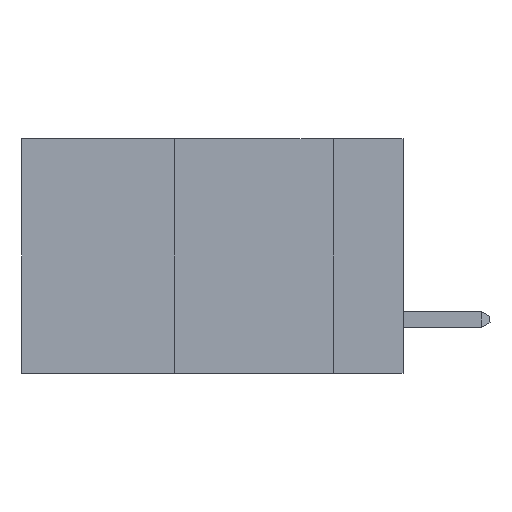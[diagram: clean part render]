
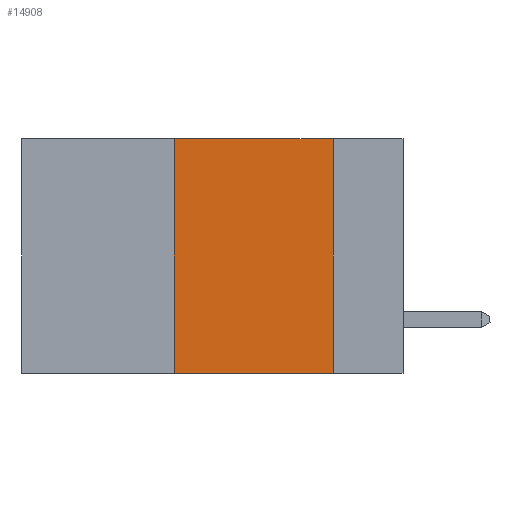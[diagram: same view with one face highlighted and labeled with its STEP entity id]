
A CAD part, left-side view. The second image highlights one B-rep face of the part: STEP entity #14908.
In plain terms, the highlighted planar face has unit normal (-1, 0, 0).
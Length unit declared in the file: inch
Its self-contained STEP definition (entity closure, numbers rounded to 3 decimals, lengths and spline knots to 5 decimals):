
#167 = AXIS2_PLACEMENT_3D ( 'NONE', #16502, #6060, #18195 ) ;
#634 = VECTOR ( 'NONE', #14794, 39.37008 ) ;
#663 = DIRECTION ( 'NONE',  ( 0., -1., 0. ) ) ;
#746 = CARTESIAN_POINT ( 'NONE',  ( 0., 0.6, -0.37 ) ) ;
#875 = ORIENTED_EDGE ( 'NONE', *, *, #21673, .F. ) ;
#2626 = VECTOR ( 'NONE', #20001, 39.37008 ) ;
#4092 = VECTOR ( 'NONE', #7222, 39.37008 ) ;
#4272 = LINE ( 'NONE', #746, #4816 ) ;
#4816 = VECTOR ( 'NONE', #663, 39.37008 ) ;
#5434 = CARTESIAN_POINT ( 'NONE',  ( 0., 0.6, 0. ) ) ;
#5677 = VERTEX_POINT ( 'NONE', #15932 ) ;
#5839 = LINE ( 'NONE', #6082, #634 ) ;
#6060 = DIRECTION ( 'NONE',  ( 1., 0., 0. ) ) ;
#6082 = CARTESIAN_POINT ( 'NONE',  ( 0., 0.36, 0. ) ) ;
#6743 = LINE ( 'NONE', #7911, #2626 ) ;
#7222 = DIRECTION ( 'NONE',  ( 0., -1., 0. ) ) ;
#7911 = CARTESIAN_POINT ( 'NONE',  ( 0., 0.11, 0. ) ) ;
#9155 = VERTEX_POINT ( 'NONE', #21210 ) ;
#10629 = VERTEX_POINT ( 'NONE', #21598 ) ;
#10779 = ORIENTED_EDGE ( 'NONE', *, *, #11926, .T. ) ;
#10820 = VERTEX_POINT ( 'NONE', #16890 ) ;
#11926 = EDGE_CURVE ( 'NONE', #9155, #10629, #4272, .T. ) ;
#14794 = DIRECTION ( 'NONE',  ( 0., 0., 1. ) ) ;
#14908 = ADVANCED_FACE ( 'NONE', ( #18569 ), #21575, .F. ) ;
#15932 = CARTESIAN_POINT ( 'NONE',  ( 0., 0.36, 0. ) ) ;
#16502 = CARTESIAN_POINT ( 'NONE',  ( 0., 0.6, 0. ) ) ;
#16565 = EDGE_CURVE ( 'NONE', #5677, #10820, #22486, .T. ) ;
#16890 = CARTESIAN_POINT ( 'NONE',  ( 0., 0.11, 0. ) ) ;
#18195 = DIRECTION ( 'NONE',  ( 0., 0., -1. ) ) ;
#18278 = ORIENTED_EDGE ( 'NONE', *, *, #20542, .F. ) ;
#18569 = FACE_OUTER_BOUND ( 'NONE', #20395, .T. ) ;
#18816 = ORIENTED_EDGE ( 'NONE', *, *, #16565, .F. ) ;
#20001 = DIRECTION ( 'NONE',  ( 0., 0., -1. ) ) ;
#20395 = EDGE_LOOP ( 'NONE', ( #18278, #18816, #875, #10779 ) ) ;
#20542 = EDGE_CURVE ( 'NONE', #10820, #10629, #6743, .T. ) ;
#21210 = CARTESIAN_POINT ( 'NONE',  ( 0., 0.36, -0.37 ) ) ;
#21575 = PLANE ( 'NONE',  #167 ) ;
#21598 = CARTESIAN_POINT ( 'NONE',  ( 0., 0.11, -0.37 ) ) ;
#21673 = EDGE_CURVE ( 'NONE', #9155, #5677, #5839, .T. ) ;
#22486 = LINE ( 'NONE', #5434, #4092 ) ;
